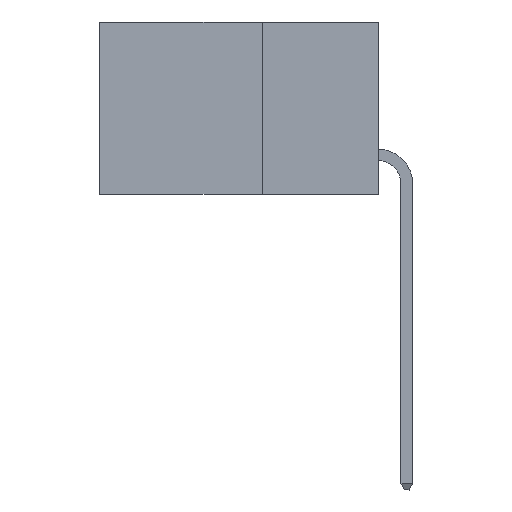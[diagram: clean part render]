
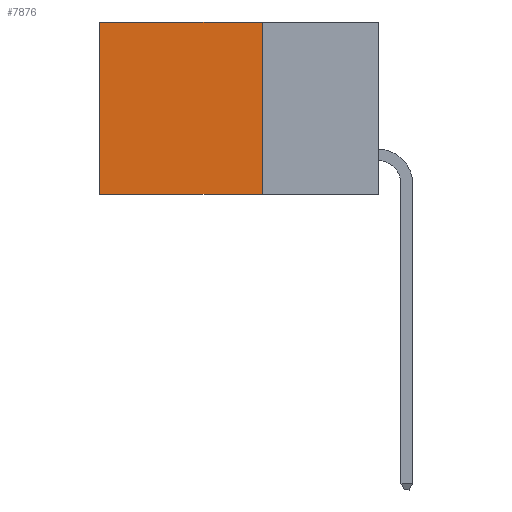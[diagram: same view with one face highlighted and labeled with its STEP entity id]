
A CAD part, left-side view. The second image highlights one B-rep face of the part: STEP entity #7876.
In plain terms, the highlighted planar face has unit normal (-1, 0, 0).
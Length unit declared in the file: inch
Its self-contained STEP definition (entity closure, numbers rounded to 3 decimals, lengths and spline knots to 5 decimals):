
#213 = DIRECTION ( 'NONE',  ( 0., 1., 0. ) ) ;
#696 = ORIENTED_EDGE ( 'NONE', *, *, #4098, .T. ) ;
#749 = EDGE_CURVE ( 'NONE', #2662, #5389, #8455, .T. ) ;
#1425 = PLANE ( 'NONE',  #2039 ) ;
#1683 = CARTESIAN_POINT ( 'NONE',  ( 0.2615, 0.25, -0.37 ) ) ;
#2039 = AXIS2_PLACEMENT_3D ( 'NONE', #9874, #5610, #8141 ) ;
#2308 = FACE_OUTER_BOUND ( 'NONE', #10018, .T. ) ;
#2351 = VERTEX_POINT ( 'NONE', #10578 ) ;
#2616 = LINE ( 'NONE', #9575, #7237 ) ;
#2662 = VERTEX_POINT ( 'NONE', #4297 ) ;
#3618 = CARTESIAN_POINT ( 'NONE',  ( 0.2615, 0.6, 0. ) ) ;
#4098 = EDGE_CURVE ( 'NONE', #2662, #5915, #6274, .T. ) ;
#4297 = CARTESIAN_POINT ( 'NONE',  ( 0.2615, 0.25, 0. ) ) ;
#5365 = DIRECTION ( 'NONE',  ( 0., 1., 0. ) ) ;
#5389 = VERTEX_POINT ( 'NONE', #7534 ) ;
#5437 = CARTESIAN_POINT ( 'NONE',  ( 0.2615, 0.6, -0.37 ) ) ;
#5503 = DIRECTION ( 'NONE',  ( 0., 0., -1. ) ) ;
#5610 = DIRECTION ( 'NONE',  ( 1., 0., 0. ) ) ;
#5611 = VECTOR ( 'NONE', #213, 39.37008 ) ;
#5744 = VECTOR ( 'NONE', #5503, 39.37008 ) ;
#5915 = VERTEX_POINT ( 'NONE', #3618 ) ;
#6274 = LINE ( 'NONE', #8625, #5611 ) ;
#6600 = ORIENTED_EDGE ( 'NONE', *, *, #8120, .F. ) ;
#6814 = DIRECTION ( 'NONE',  ( 0., 0., -1. ) ) ;
#7237 = VECTOR ( 'NONE', #5365, 39.37008 ) ;
#7534 = CARTESIAN_POINT ( 'NONE',  ( 0.2615, 0.25, -0.37 ) ) ;
#7640 = ORIENTED_EDGE ( 'NONE', *, *, #749, .F. ) ;
#7795 = EDGE_CURVE ( 'NONE', #5915, #2351, #10785, .T. ) ;
#7876 = ADVANCED_FACE ( 'NONE', ( #2308 ), #1425, .F. ) ;
#8120 = EDGE_CURVE ( 'NONE', #5389, #2351, #2616, .T. ) ;
#8141 = DIRECTION ( 'NONE',  ( 0., 0., -1. ) ) ;
#8455 = LINE ( 'NONE', #1683, #10835 ) ;
#8625 = CARTESIAN_POINT ( 'NONE',  ( 0.2615, 0.25, 0. ) ) ;
#9575 = CARTESIAN_POINT ( 'NONE',  ( 0.2615, 0.25, -0.37 ) ) ;
#9874 = CARTESIAN_POINT ( 'NONE',  ( 0.2615, 0.25, -0.37 ) ) ;
#10018 = EDGE_LOOP ( 'NONE', ( #10849, #6600, #7640, #696 ) ) ;
#10578 = CARTESIAN_POINT ( 'NONE',  ( 0.2615, 0.6, -0.37 ) ) ;
#10785 = LINE ( 'NONE', #5437, #5744 ) ;
#10835 = VECTOR ( 'NONE', #6814, 39.37008 ) ;
#10849 = ORIENTED_EDGE ( 'NONE', *, *, #7795, .T. ) ;
